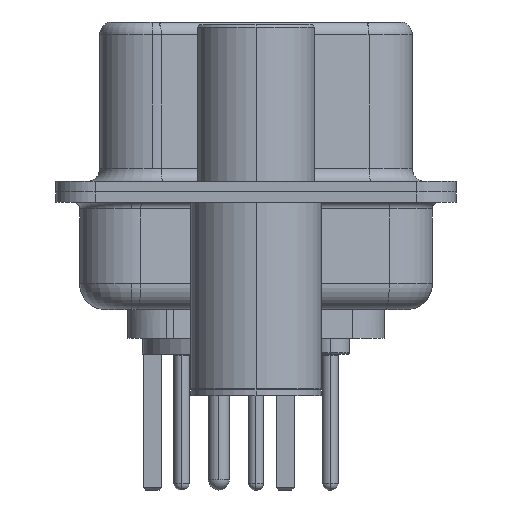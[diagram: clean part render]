
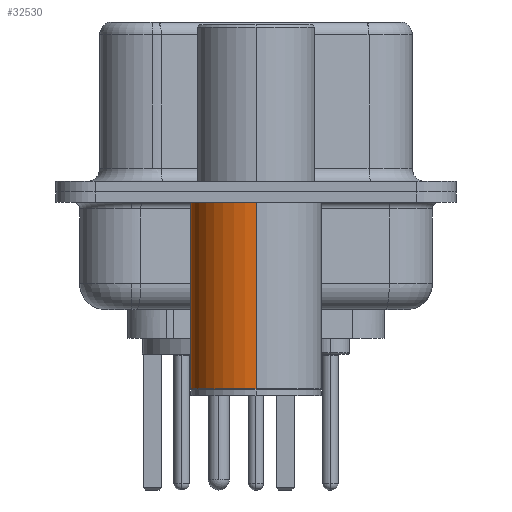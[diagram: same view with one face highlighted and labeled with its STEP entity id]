
A CAD part, left-side view. The second image highlights one B-rep face of the part: STEP entity #32530.
In plain terms, the highlighted cylindrical face has radius 2.5 mm (diameter 5 mm), a partial arc.
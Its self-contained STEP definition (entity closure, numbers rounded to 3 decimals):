
#47 = VERTEX_POINT ( 'NONE', #32752 ) ;
#3017 = CYLINDRICAL_SURFACE ( 'NONE', #27853, 2.5 ) ;
#5342 = VERTEX_POINT ( 'NONE', #20210 ) ;
#6713 = DIRECTION ( 'NONE',  ( 0., 0., 1. ) ) ;
#7206 = AXIS2_PLACEMENT_3D ( 'NONE', #32437, #15857, #35223 ) ;
#7300 = CARTESIAN_POINT ( 'NONE',  ( -2.5, 0., -0.4 ) ) ;
#9138 = ORIENTED_EDGE ( 'NONE', *, *, #30595, .F. ) ;
#10703 = DIRECTION ( 'NONE',  ( 0., 0., 1. ) ) ;
#11117 = CARTESIAN_POINT ( 'NONE',  ( -2.5, 0., -7.525 ) ) ;
#11665 = VECTOR ( 'NONE', #26612, 1000. ) ;
#11790 = VERTEX_POINT ( 'NONE', #11117 ) ;
#12123 = CARTESIAN_POINT ( 'NONE',  ( 2.5, 0., 0.581 ) ) ;
#13876 = EDGE_CURVE ( 'NONE', #47, #17573, #27464, .T. ) ;
#14906 = VECTOR ( 'NONE', #25995, 1000. ) ;
#15547 = EDGE_LOOP ( 'NONE', ( #29754, #27007, #17354, #9138 ) ) ;
#15759 = LINE ( 'NONE', #12123, #14906 ) ;
#15857 = DIRECTION ( 'NONE',  ( 0., 0., 1. ) ) ;
#17354 = ORIENTED_EDGE ( 'NONE', *, *, #13876, .F. ) ;
#17573 = VERTEX_POINT ( 'NONE', #7300 ) ;
#19087 = LINE ( 'NONE', #34903, #11665 ) ;
#20210 = CARTESIAN_POINT ( 'NONE',  ( 2.5, 0., -7.525 ) ) ;
#21937 = CIRCLE ( 'NONE', #26033, 2.5 ) ;
#23412 = CARTESIAN_POINT ( 'NONE',  ( 0., 0., -7.525 ) ) ;
#24055 = EDGE_CURVE ( 'NONE', #11790, #17573, #19087, .T. ) ;
#24613 = CARTESIAN_POINT ( 'NONE',  ( 0., 0., 0.581 ) ) ;
#25995 = DIRECTION ( 'NONE',  ( 0., 0., 1. ) ) ;
#26033 = AXIS2_PLACEMENT_3D ( 'NONE', #23412, #6713, #26153 ) ;
#26153 = DIRECTION ( 'NONE',  ( 1., 0., 0. ) ) ;
#26612 = DIRECTION ( 'NONE',  ( 0., 0., 1. ) ) ;
#27007 = ORIENTED_EDGE ( 'NONE', *, *, #24055, .T. ) ;
#27464 = CIRCLE ( 'NONE', #7206, 2.5 ) ;
#27853 = AXIS2_PLACEMENT_3D ( 'NONE', #24613, #10703, #35659 ) ;
#29754 = ORIENTED_EDGE ( 'NONE', *, *, #35771, .T. ) ;
#30595 = EDGE_CURVE ( 'NONE', #5342, #47, #15759, .T. ) ;
#32437 = CARTESIAN_POINT ( 'NONE',  ( 0., 0., -0.4 ) ) ;
#32521 = FACE_OUTER_BOUND ( 'NONE', #15547, .T. ) ;
#32530 = ADVANCED_FACE ( 'NONE', ( #32521 ), #3017, .T. ) ;
#32752 = CARTESIAN_POINT ( 'NONE',  ( 2.5, 0., -0.4 ) ) ;
#34903 = CARTESIAN_POINT ( 'NONE',  ( -2.5, 0., 0.581 ) ) ;
#35223 = DIRECTION ( 'NONE',  ( 1., 0., 0. ) ) ;
#35659 = DIRECTION ( 'NONE',  ( 1., 0., 0. ) ) ;
#35771 = EDGE_CURVE ( 'NONE', #5342, #11790, #21937, .T. ) ;
